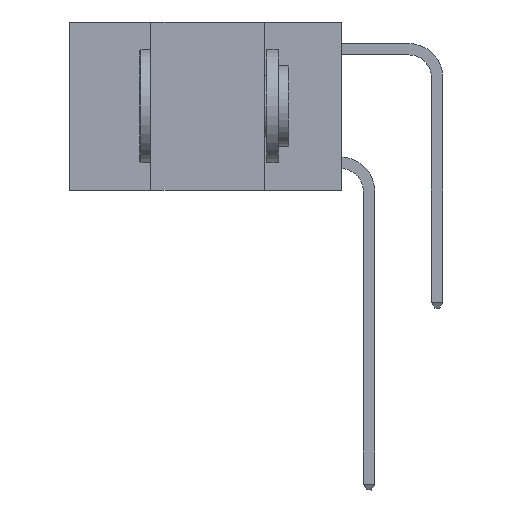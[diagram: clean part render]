
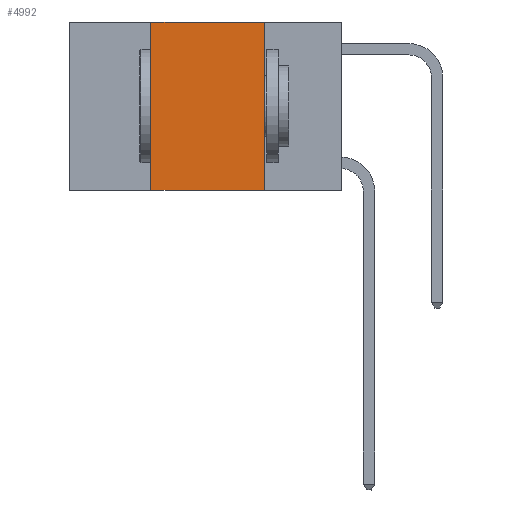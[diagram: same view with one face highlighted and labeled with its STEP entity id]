
A CAD part, left-side view. The second image highlights one B-rep face of the part: STEP entity #4992.
In plain terms, the highlighted planar face has unit normal (-1, 0, 0).
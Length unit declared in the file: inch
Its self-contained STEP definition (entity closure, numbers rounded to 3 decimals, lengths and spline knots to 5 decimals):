
#51 = ORIENTED_EDGE ( 'NONE', *, *, #12868, .F. ) ;
#364 = DIRECTION ( 'NONE',  ( 0., 0., -1. ) ) ;
#1779 = EDGE_CURVE ( 'NONE', #4902, #18838, #18195, .T. ) ;
#1889 = CARTESIAN_POINT ( 'NONE',  ( 0., 0.42, -0.37 ) ) ;
#1920 = ORIENTED_EDGE ( 'NONE', *, *, #8393, .T. ) ;
#2217 = FACE_OUTER_BOUND ( 'NONE', #20302, .T. ) ;
#2955 = ORIENTED_EDGE ( 'NONE', *, *, #1779, .F. ) ;
#3258 = AXIS2_PLACEMENT_3D ( 'NONE', #11779, #10309, #364 ) ;
#3629 = VERTEX_POINT ( 'NONE', #14553 ) ;
#4902 = VERTEX_POINT ( 'NONE', #16508 ) ;
#4992 = ADVANCED_FACE ( 'NONE', ( #2217 ), #19983, .F. ) ;
#5742 = DIRECTION ( 'NONE',  ( 0., -1., 0. ) ) ;
#5780 = LINE ( 'NONE', #15477, #13918 ) ;
#6028 = LINE ( 'NONE', #16096, #13141 ) ;
#6188 = VERTEX_POINT ( 'NONE', #1889 ) ;
#8393 = EDGE_CURVE ( 'NONE', #6188, #18838, #5780, .T. ) ;
#8636 = EDGE_CURVE ( 'NONE', #6188, #3629, #6028, .T. ) ;
#9246 = DIRECTION ( 'NONE',  ( 0., 0., -1. ) ) ;
#10166 = VECTOR ( 'NONE', #16780, 39.37008 ) ;
#10309 = DIRECTION ( 'NONE',  ( 1., 0., 0. ) ) ;
#11779 = CARTESIAN_POINT ( 'NONE',  ( 0., 0.6, 0. ) ) ;
#12868 = EDGE_CURVE ( 'NONE', #3629, #4902, #14460, .T. ) ;
#13141 = VECTOR ( 'NONE', #17753, 39.37008 ) ;
#13190 = ORIENTED_EDGE ( 'NONE', *, *, #8636, .F. ) ;
#13890 = VECTOR ( 'NONE', #9246, 39.37008 ) ;
#13918 = VECTOR ( 'NONE', #5742, 39.37008 ) ;
#14460 = LINE ( 'NONE', #15143, #10166 ) ;
#14553 = CARTESIAN_POINT ( 'NONE',  ( 0., 0.42, 0. ) ) ;
#15143 = CARTESIAN_POINT ( 'NONE',  ( 0., 0.6, 0. ) ) ;
#15278 = CARTESIAN_POINT ( 'NONE',  ( 0., 0.17, -0.37 ) ) ;
#15477 = CARTESIAN_POINT ( 'NONE',  ( 0., 0.6, -0.37 ) ) ;
#16096 = CARTESIAN_POINT ( 'NONE',  ( 0., 0.42, 0. ) ) ;
#16508 = CARTESIAN_POINT ( 'NONE',  ( 0., 0.17, 0. ) ) ;
#16780 = DIRECTION ( 'NONE',  ( 0., -1., 0. ) ) ;
#17753 = DIRECTION ( 'NONE',  ( 0., 0., 1. ) ) ;
#18195 = LINE ( 'NONE', #20969, #13890 ) ;
#18838 = VERTEX_POINT ( 'NONE', #15278 ) ;
#19983 = PLANE ( 'NONE',  #3258 ) ;
#20302 = EDGE_LOOP ( 'NONE', ( #2955, #51, #13190, #1920 ) ) ;
#20969 = CARTESIAN_POINT ( 'NONE',  ( 0., 0.17, 0. ) ) ;
